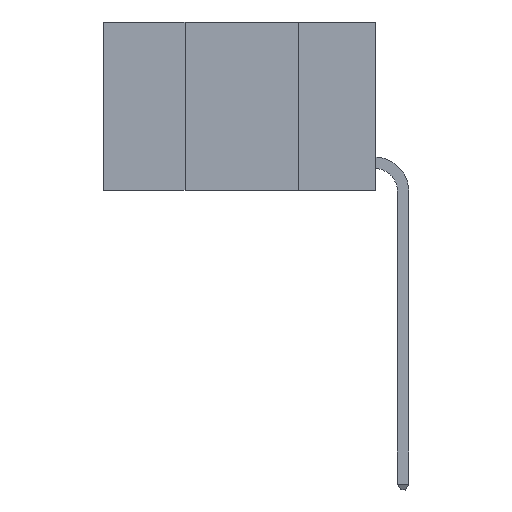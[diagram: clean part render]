
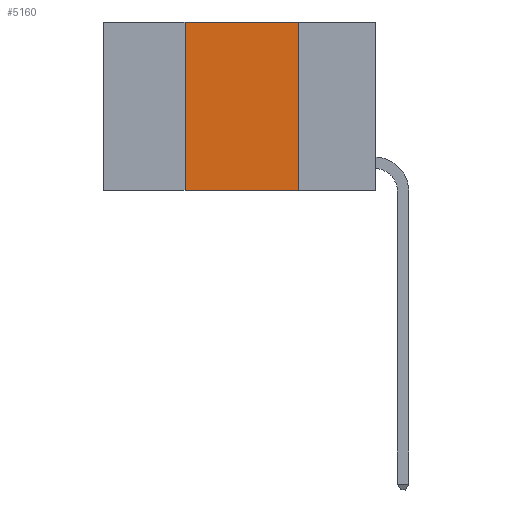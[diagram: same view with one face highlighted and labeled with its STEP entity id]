
A CAD part, left-side view. The second image highlights one B-rep face of the part: STEP entity #5160.
In plain terms, the highlighted planar face has unit normal (-1, 0, 0).
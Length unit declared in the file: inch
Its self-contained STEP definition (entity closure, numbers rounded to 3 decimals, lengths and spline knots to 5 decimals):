
#122 = LINE ( 'NONE', #8296, #3703 ) ;
#1380 = VERTEX_POINT ( 'NONE', #7787 ) ;
#2330 = EDGE_CURVE ( 'NONE', #1380, #9238, #10528, .T. ) ;
#2780 = DIRECTION ( 'NONE',  ( 0., -1., 0. ) ) ;
#3135 = CARTESIAN_POINT ( 'NONE',  ( 0., 0.17, 0. ) ) ;
#3703 = VECTOR ( 'NONE', #22259, 39.37008 ) ;
#4248 = CARTESIAN_POINT ( 'NONE',  ( 0., 0.6, 0. ) ) ;
#5160 = ADVANCED_FACE ( 'NONE', ( #18930 ), #14899, .F. ) ;
#7787 = CARTESIAN_POINT ( 'NONE',  ( 0., 0.42, 0. ) ) ;
#8296 = CARTESIAN_POINT ( 'NONE',  ( 0., 0.42, 0. ) ) ;
#9238 = VERTEX_POINT ( 'NONE', #3135 ) ;
#10528 = LINE ( 'NONE', #4248, #15291 ) ;
#10751 = DIRECTION ( 'NONE',  ( 0., 0., -1. ) ) ;
#11099 = CARTESIAN_POINT ( 'NONE',  ( 0., 0.6, -0.37 ) ) ;
#11930 = ORIENTED_EDGE ( 'NONE', *, *, #25439, .F. ) ;
#12683 = ORIENTED_EDGE ( 'NONE', *, *, #16442, .T. ) ;
#13028 = DIRECTION ( 'NONE',  ( 1., 0., 0. ) ) ;
#13208 = DIRECTION ( 'NONE',  ( 0., 0., -1. ) ) ;
#14071 = VECTOR ( 'NONE', #13208, 39.37008 ) ;
#14428 = EDGE_CURVE ( 'NONE', #9238, #15128, #19372, .T. ) ;
#14730 = LINE ( 'NONE', #11099, #24011 ) ;
#14899 = PLANE ( 'NONE',  #18543 ) ;
#15035 = ORIENTED_EDGE ( 'NONE', *, *, #2330, .F. ) ;
#15128 = VERTEX_POINT ( 'NONE', #24437 ) ;
#15291 = VECTOR ( 'NONE', #16835, 39.37008 ) ;
#16442 = EDGE_CURVE ( 'NONE', #17488, #15128, #14730, .T. ) ;
#16835 = DIRECTION ( 'NONE',  ( 0., -1., 0. ) ) ;
#17090 = CARTESIAN_POINT ( 'NONE',  ( 0., 0.17, 0. ) ) ;
#17488 = VERTEX_POINT ( 'NONE', #25640 ) ;
#17665 = CARTESIAN_POINT ( 'NONE',  ( 0., 0.6, 0. ) ) ;
#18543 = AXIS2_PLACEMENT_3D ( 'NONE', #17665, #13028, #10751 ) ;
#18832 = ORIENTED_EDGE ( 'NONE', *, *, #14428, .F. ) ;
#18930 = FACE_OUTER_BOUND ( 'NONE', #21428, .T. ) ;
#19372 = LINE ( 'NONE', #17090, #14071 ) ;
#21428 = EDGE_LOOP ( 'NONE', ( #18832, #15035, #11930, #12683 ) ) ;
#22259 = DIRECTION ( 'NONE',  ( 0., 0., 1. ) ) ;
#24011 = VECTOR ( 'NONE', #2780, 39.37008 ) ;
#24437 = CARTESIAN_POINT ( 'NONE',  ( 0., 0.17, -0.37 ) ) ;
#25439 = EDGE_CURVE ( 'NONE', #17488, #1380, #122, .T. ) ;
#25640 = CARTESIAN_POINT ( 'NONE',  ( 0., 0.42, -0.37 ) ) ;
